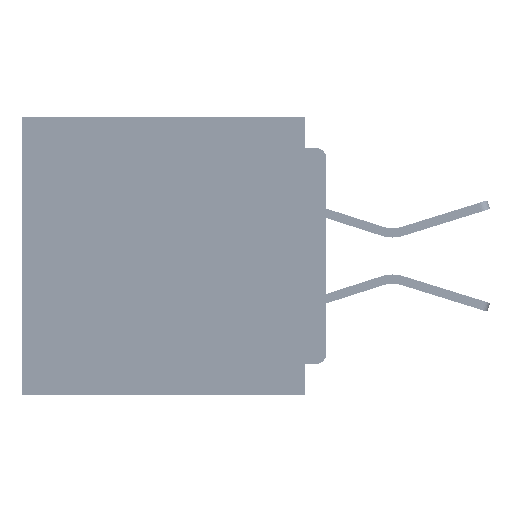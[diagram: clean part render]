
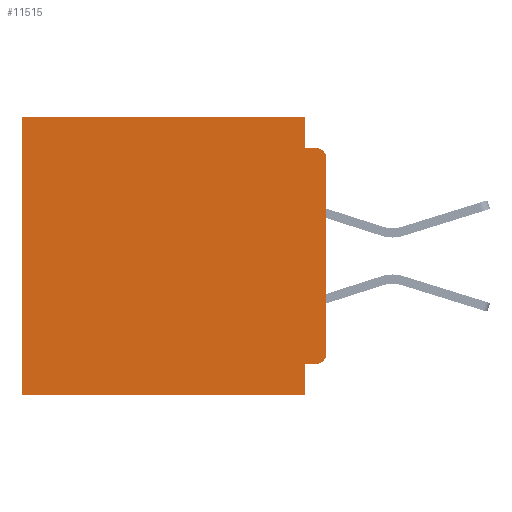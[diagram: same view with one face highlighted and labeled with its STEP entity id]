
A CAD part, left-side view. The second image highlights one B-rep face of the part: STEP entity #11515.
In plain terms, the highlighted planar face has unit normal (-1, 0, 0).
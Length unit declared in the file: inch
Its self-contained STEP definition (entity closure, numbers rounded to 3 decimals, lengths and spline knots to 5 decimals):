
#99 = EDGE_CURVE ( 'NONE', #4105, #31018, #43722, .T. ) ;
#525 = ORIENTED_EDGE ( 'NONE', *, *, #22089, .T. ) ;
#1110 = LINE ( 'NONE', #20317, #26241 ) ;
#2922 = VERTEX_POINT ( 'NONE', #16623 ) ;
#3745 = VERTEX_POINT ( 'NONE', #39737 ) ;
#4105 = VERTEX_POINT ( 'NONE', #32415 ) ;
#5547 = AXIS2_PLACEMENT_3D ( 'NONE', #45597, #20728, #55610 ) ;
#6096 = CARTESIAN_POINT ( 'NONE',  ( 0.3, 0., -0.355 ) ) ;
#6486 = ORIENTED_EDGE ( 'NONE', *, *, #49749, .F. ) ;
#7382 = VECTOR ( 'NONE', #60828, 39.37008 ) ;
#7492 = VERTEX_POINT ( 'NONE', #12734 ) ;
#8513 = VERTEX_POINT ( 'NONE', #30338 ) ;
#9669 = CARTESIAN_POINT ( 'NONE',  ( 0.3, 0.015, -0.34 ) ) ;
#10621 = VERTEX_POINT ( 'NONE', #33548 ) ;
#10932 = EDGE_CURVE ( 'NONE', #4105, #7492, #26733, .T. ) ;
#10973 = VECTOR ( 'NONE', #34920, 39.37008 ) ;
#11170 = DIRECTION ( 'NONE',  ( 0., 1., 0. ) ) ;
#11515 = ADVANCED_FACE ( 'NONE', ( #29868 ), #15699, .F. ) ;
#12346 = ORIENTED_EDGE ( 'NONE', *, *, #99, .T. ) ;
#12387 = EDGE_CURVE ( 'NONE', #7492, #3745, #23775, .T. ) ;
#12637 = VERTEX_POINT ( 'NONE', #28914 ) ;
#12734 = CARTESIAN_POINT ( 'NONE',  ( 0.3, 0.031, -0.355 ) ) ;
#13414 = VECTOR ( 'NONE', #11170, 39.37008 ) ;
#13632 = EDGE_LOOP ( 'NONE', ( #25324, #23059, #6486, #41145, #525, #20089, #25852, #55598, #23851, #12346 ) ) ;
#14085 = CARTESIAN_POINT ( 'NONE',  ( 0.3, 0.015, -0.06 ) ) ;
#15010 = CARTESIAN_POINT ( 'NONE',  ( 0.3, 0.437, -0.4 ) ) ;
#15283 = DIRECTION ( 'NONE',  ( 0., 1., 0. ) ) ;
#15380 = VECTOR ( 'NONE', #48531, 39.37008 ) ;
#15699 = PLANE ( 'NONE',  #5547 ) ;
#16623 = CARTESIAN_POINT ( 'NONE',  ( 0.3, 0.031, 0. ) ) ;
#16821 = VECTOR ( 'NONE', #34723, 39.37008 ) ;
#18399 = LINE ( 'NONE', #39688, #16821 ) ;
#18529 = LINE ( 'NONE', #28737, #15380 ) ;
#19124 = DIRECTION ( 'NONE',  ( 0., 0., -1. ) ) ;
#19989 = CARTESIAN_POINT ( 'NONE',  ( 0.3, 0., -0.34 ) ) ;
#20089 = ORIENTED_EDGE ( 'NONE', *, *, #52081, .T. ) ;
#20317 = CARTESIAN_POINT ( 'NONE',  ( 0.3, 0., 0. ) ) ;
#20728 = DIRECTION ( 'NONE',  ( 1., 0., 0. ) ) ;
#20935 = CARTESIAN_POINT ( 'NONE',  ( 0.3, 0., -0.045 ) ) ;
#22089 = EDGE_CURVE ( 'NONE', #2922, #8513, #1110, .T. ) ;
#23059 = ORIENTED_EDGE ( 'NONE', *, *, #42039, .T. ) ;
#23405 = CARTESIAN_POINT ( 'NONE',  ( 0.3, 0., -0.4 ) ) ;
#23546 = EDGE_CURVE ( 'NONE', #3745, #52515, #56407, .T. ) ;
#23775 = LINE ( 'NONE', #36780, #61912 ) ;
#23851 = ORIENTED_EDGE ( 'NONE', *, *, #10932, .F. ) ;
#25324 = ORIENTED_EDGE ( 'NONE', *, *, #41519, .F. ) ;
#25504 = CARTESIAN_POINT ( 'NONE',  ( 0.3, 0.437, -0.4 ) ) ;
#25852 = ORIENTED_EDGE ( 'NONE', *, *, #23546, .F. ) ;
#26241 = VECTOR ( 'NONE', #15283, 39.37008 ) ;
#26733 = LINE ( 'NONE', #6096, #13414 ) ;
#26758 = AXIS2_PLACEMENT_3D ( 'NONE', #9669, #58273, #33494 ) ;
#28435 = DIRECTION ( 'NONE',  ( 0., 1., 0. ) ) ;
#28737 = CARTESIAN_POINT ( 'NONE',  ( 0.3, 0.031, 0. ) ) ;
#28914 = CARTESIAN_POINT ( 'NONE',  ( 0.3, 0.015, -0.045 ) ) ;
#29868 = FACE_OUTER_BOUND ( 'NONE', #13632, .T. ) ;
#30338 = CARTESIAN_POINT ( 'NONE',  ( 0.3, 0.437, 0. ) ) ;
#31018 = VERTEX_POINT ( 'NONE', #19989 ) ;
#32415 = CARTESIAN_POINT ( 'NONE',  ( 0.3, 0.015, -0.355 ) ) ;
#33223 = EDGE_CURVE ( 'NONE', #2922, #10621, #18529, .T. ) ;
#33494 = DIRECTION ( 'NONE',  ( 0., 0., -1. ) ) ;
#33548 = CARTESIAN_POINT ( 'NONE',  ( 0.3, 0.031, -0.045 ) ) ;
#34723 = DIRECTION ( 'NONE',  ( 0., 0., -1. ) ) ;
#34920 = DIRECTION ( 'NONE',  ( 0., 0., -1. ) ) ;
#36780 = CARTESIAN_POINT ( 'NONE',  ( 0.3, 0.031, -0.4 ) ) ;
#39688 = CARTESIAN_POINT ( 'NONE',  ( 0.3, 0., -0.4 ) ) ;
#39737 = CARTESIAN_POINT ( 'NONE',  ( 0.3, 0.031, -0.4 ) ) ;
#41145 = ORIENTED_EDGE ( 'NONE', *, *, #33223, .F. ) ;
#41519 = EDGE_CURVE ( 'NONE', #54740, #31018, #18399, .T. ) ;
#41762 = DIRECTION ( 'NONE',  ( 0., 0., -1. ) ) ;
#42039 = EDGE_CURVE ( 'NONE', #54740, #12637, #59600, .T. ) ;
#43190 = VECTOR ( 'NONE', #28435, 39.37008 ) ;
#43722 = CIRCLE ( 'NONE', #26758, 0.015 ) ;
#45597 = CARTESIAN_POINT ( 'NONE',  ( 0.3, 0., -0.4 ) ) ;
#48531 = DIRECTION ( 'NONE',  ( 0., 0., -1. ) ) ;
#48973 = DIRECTION ( 'NONE',  ( -1., 0., 0. ) ) ;
#49522 = AXIS2_PLACEMENT_3D ( 'NONE', #14085, #48973, #19124 ) ;
#49749 = EDGE_CURVE ( 'NONE', #10621, #12637, #60476, .T. ) ;
#52081 = EDGE_CURVE ( 'NONE', #8513, #52515, #64015, .T. ) ;
#52515 = VERTEX_POINT ( 'NONE', #25504 ) ;
#53758 = CARTESIAN_POINT ( 'NONE',  ( 0.3, 0., -0.06 ) ) ;
#54740 = VERTEX_POINT ( 'NONE', #53758 ) ;
#55598 = ORIENTED_EDGE ( 'NONE', *, *, #12387, .F. ) ;
#55610 = DIRECTION ( 'NONE',  ( 0., 0., -1. ) ) ;
#56407 = LINE ( 'NONE', #23405, #43190 ) ;
#58273 = DIRECTION ( 'NONE',  ( -1., 0., 0. ) ) ;
#59600 = CIRCLE ( 'NONE', #49522, 0.015 ) ;
#60476 = LINE ( 'NONE', #20935, #7382 ) ;
#60828 = DIRECTION ( 'NONE',  ( 0., -1., 0. ) ) ;
#61912 = VECTOR ( 'NONE', #41762, 39.37008 ) ;
#64015 = LINE ( 'NONE', #15010, #10973 ) ;
